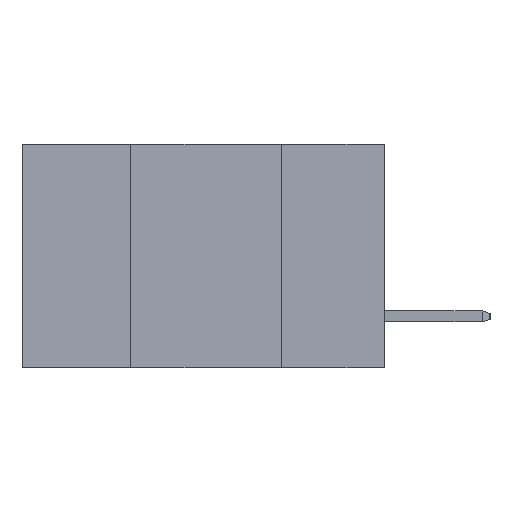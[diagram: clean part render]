
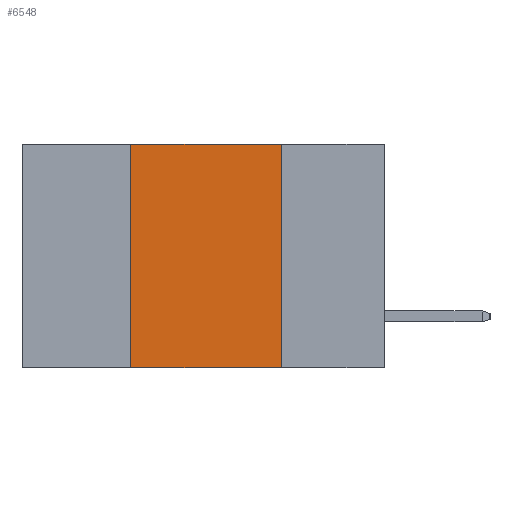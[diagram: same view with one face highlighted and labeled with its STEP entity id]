
A CAD part, left-side view. The second image highlights one B-rep face of the part: STEP entity #6548.
In plain terms, the highlighted planar face has unit normal (-1, 0, 0).
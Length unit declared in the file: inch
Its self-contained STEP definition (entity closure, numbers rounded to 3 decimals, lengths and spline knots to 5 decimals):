
#875 = DIRECTION ( 'NONE',  ( 0., 0., -1. ) ) ;
#1351 = ORIENTED_EDGE ( 'NONE', *, *, #7679, .F. ) ;
#1386 = CARTESIAN_POINT ( 'NONE',  ( 0., 0.42, -0.37 ) ) ;
#1847 = CARTESIAN_POINT ( 'NONE',  ( 0., 0.42, -0.37 ) ) ;
#2174 = PLANE ( 'NONE',  #4056 ) ;
#2365 = VECTOR ( 'NONE', #2948, 39.37008 ) ;
#2697 = LINE ( 'NONE', #1847, #2365 ) ;
#2775 = VECTOR ( 'NONE', #875, 39.37008 ) ;
#2948 = DIRECTION ( 'NONE',  ( 0., 0., 1. ) ) ;
#3564 = ORIENTED_EDGE ( 'NONE', *, *, #9508, .F. ) ;
#4056 = AXIS2_PLACEMENT_3D ( 'NONE', #10612, #4325, #11625 ) ;
#4185 = LINE ( 'NONE', #10974, #6656 ) ;
#4200 = ORIENTED_EDGE ( 'NONE', *, *, #8651, .T. ) ;
#4264 = LINE ( 'NONE', #10579, #6737 ) ;
#4325 = DIRECTION ( 'NONE',  ( 1., 0., 0. ) ) ;
#5583 = LINE ( 'NONE', #7251, #2775 ) ;
#5956 = EDGE_CURVE ( 'NONE', #9417, #7992, #4264, .T. ) ;
#6120 = VERTEX_POINT ( 'NONE', #1386 ) ;
#6322 = ORIENTED_EDGE ( 'NONE', *, *, #5956, .F. ) ;
#6548 = ADVANCED_FACE ( 'NONE', ( #13340 ), #2174, .F. ) ;
#6656 = VECTOR ( 'NONE', #11990, 39.37008 ) ;
#6737 = VECTOR ( 'NONE', #10622, 39.37008 ) ;
#7251 = CARTESIAN_POINT ( 'NONE',  ( 0., 0.17, -0.37 ) ) ;
#7679 = EDGE_CURVE ( 'NONE', #6120, #9417, #2697, .T. ) ;
#7992 = VERTEX_POINT ( 'NONE', #12760 ) ;
#8651 = EDGE_CURVE ( 'NONE', #6120, #12790, #4185, .T. ) ;
#9417 = VERTEX_POINT ( 'NONE', #11204 ) ;
#9508 = EDGE_CURVE ( 'NONE', #7992, #12790, #5583, .T. ) ;
#10579 = CARTESIAN_POINT ( 'NONE',  ( 0., 0.6, 0. ) ) ;
#10612 = CARTESIAN_POINT ( 'NONE',  ( 0., 0.6, 0. ) ) ;
#10622 = DIRECTION ( 'NONE',  ( 0., -1., 0. ) ) ;
#10974 = CARTESIAN_POINT ( 'NONE',  ( 0., 0.6, -0.37 ) ) ;
#11204 = CARTESIAN_POINT ( 'NONE',  ( 0., 0.42, 0. ) ) ;
#11625 = DIRECTION ( 'NONE',  ( 0., 0., -1. ) ) ;
#11990 = DIRECTION ( 'NONE',  ( 0., -1., 0. ) ) ;
#12675 = CARTESIAN_POINT ( 'NONE',  ( 0., 0.17, -0.37 ) ) ;
#12760 = CARTESIAN_POINT ( 'NONE',  ( 0., 0.17, 0. ) ) ;
#12790 = VERTEX_POINT ( 'NONE', #12675 ) ;
#13070 = EDGE_LOOP ( 'NONE', ( #3564, #6322, #1351, #4200 ) ) ;
#13340 = FACE_OUTER_BOUND ( 'NONE', #13070, .T. ) ;
